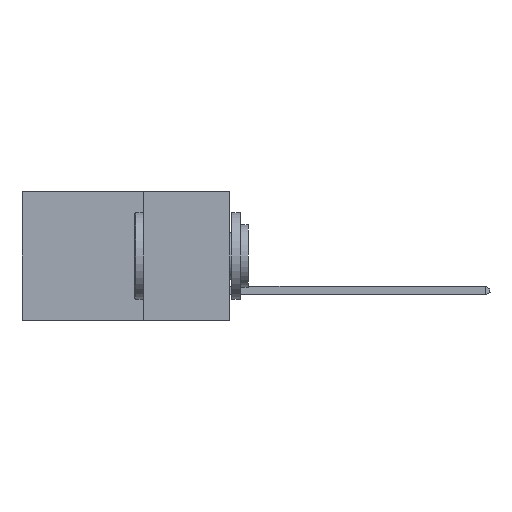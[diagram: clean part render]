
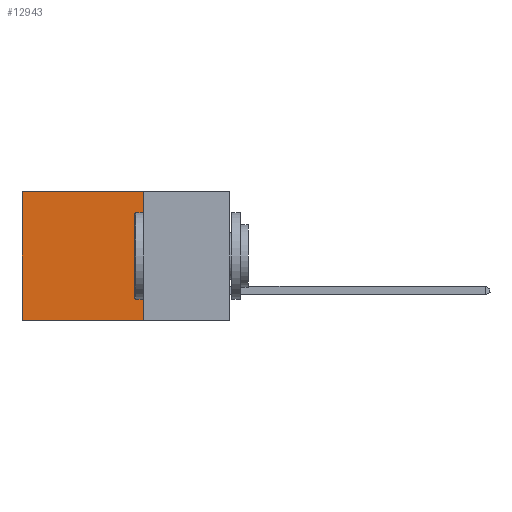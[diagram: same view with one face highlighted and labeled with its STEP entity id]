
A CAD part, left-side view. The second image highlights one B-rep face of the part: STEP entity #12943.
In plain terms, the highlighted planar face has unit normal (-1, 0, 0).
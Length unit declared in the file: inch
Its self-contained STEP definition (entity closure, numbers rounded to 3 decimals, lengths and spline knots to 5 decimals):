
#992 = DIRECTION ( 'NONE',  ( 0., 1., 0. ) ) ;
#1126 = DIRECTION ( 'NONE',  ( 0., 0., -1. ) ) ;
#1696 = EDGE_CURVE ( 'NONE', #16313, #23016, #19254, .T. ) ;
#2514 = VECTOR ( 'NONE', #5222, 39.37008 ) ;
#2976 = CARTESIAN_POINT ( 'NONE',  ( 0.298, 0.25, 0. ) ) ;
#4878 = CARTESIAN_POINT ( 'NONE',  ( 0.298, 0.6, 0. ) ) ;
#5222 = DIRECTION ( 'NONE',  ( 0., 1., 0. ) ) ;
#6306 = ORIENTED_EDGE ( 'NONE', *, *, #14540, .F. ) ;
#6469 = ORIENTED_EDGE ( 'NONE', *, *, #14386, .T. ) ;
#8064 = DIRECTION ( 'NONE',  ( 0., 0., -1. ) ) ;
#10116 = PLANE ( 'NONE',  #18160 ) ;
#10596 = EDGE_LOOP ( 'NONE', ( #16129, #14169, #6306, #6469 ) ) ;
#11113 = CARTESIAN_POINT ( 'NONE',  ( 0.298, 0.6, -0.37 ) ) ;
#11335 = CARTESIAN_POINT ( 'NONE',  ( 0.298, 0.25, -0.37 ) ) ;
#12499 = DIRECTION ( 'NONE',  ( 0., 0., -1. ) ) ;
#12943 = ADVANCED_FACE ( 'NONE', ( #14077 ), #10116, .F. ) ;
#13334 = LINE ( 'NONE', #24032, #17525 ) ;
#13348 = LINE ( 'NONE', #2976, #15778 ) ;
#14077 = FACE_OUTER_BOUND ( 'NONE', #10596, .T. ) ;
#14167 = VECTOR ( 'NONE', #12499, 39.37008 ) ;
#14169 = ORIENTED_EDGE ( 'NONE', *, *, #15771, .F. ) ;
#14386 = EDGE_CURVE ( 'NONE', #24040, #16313, #17886, .T. ) ;
#14540 = EDGE_CURVE ( 'NONE', #24040, #14917, #13348, .T. ) ;
#14917 = VERTEX_POINT ( 'NONE', #11335 ) ;
#15564 = CARTESIAN_POINT ( 'NONE',  ( 0.298, 0.6, 0. ) ) ;
#15771 = EDGE_CURVE ( 'NONE', #14917, #23016, #13334, .T. ) ;
#15778 = VECTOR ( 'NONE', #1126, 39.37008 ) ;
#16129 = ORIENTED_EDGE ( 'NONE', *, *, #1696, .T. ) ;
#16313 = VERTEX_POINT ( 'NONE', #15564 ) ;
#16792 = CARTESIAN_POINT ( 'NONE',  ( 0.298, 0.25, 0. ) ) ;
#17525 = VECTOR ( 'NONE', #992, 39.37008 ) ;
#17886 = LINE ( 'NONE', #16792, #2514 ) ;
#17934 = CARTESIAN_POINT ( 'NONE',  ( 0.298, 0.25, 0. ) ) ;
#18160 = AXIS2_PLACEMENT_3D ( 'NONE', #17934, #21538, #8064 ) ;
#19254 = LINE ( 'NONE', #4878, #14167 ) ;
#19782 = CARTESIAN_POINT ( 'NONE',  ( 0.298, 0.25, 0. ) ) ;
#21538 = DIRECTION ( 'NONE',  ( 1., 0., 0. ) ) ;
#23016 = VERTEX_POINT ( 'NONE', #11113 ) ;
#24032 = CARTESIAN_POINT ( 'NONE',  ( 0.298, 0.25, -0.37 ) ) ;
#24040 = VERTEX_POINT ( 'NONE', #19782 ) ;
